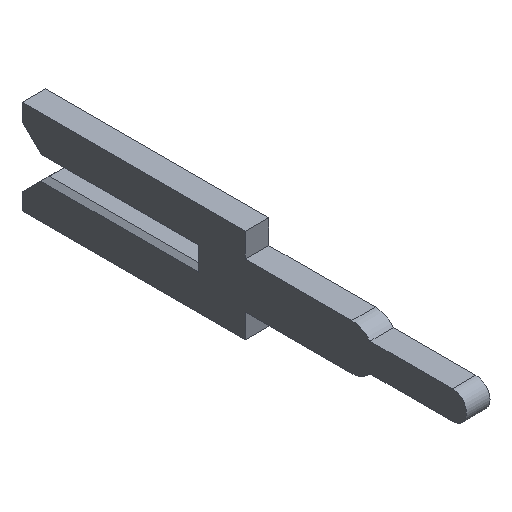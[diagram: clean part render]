
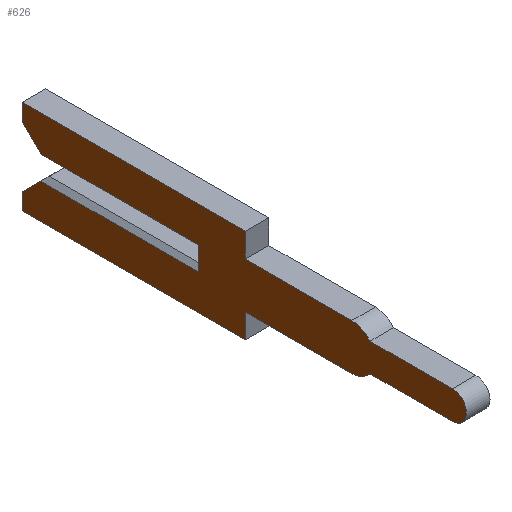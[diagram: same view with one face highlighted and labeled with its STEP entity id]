
A CAD part, isometric view. The second image highlights one B-rep face of the part: STEP entity #626.
In plain terms, the highlighted planar face has unit normal (-1, 0, 0).
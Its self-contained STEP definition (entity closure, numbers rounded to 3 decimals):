
#2 = VERTEX_POINT ( 'NONE', #481 ) ;
#6 = PLANE ( 'NONE',  #403 ) ;
#7 = VERTEX_POINT ( 'NONE', #49 ) ;
#17 = EDGE_CURVE ( 'NONE', #131, #633, #643, .T. ) ;
#24 = VECTOR ( 'NONE', #287, 1000. ) ;
#26 = DIRECTION ( 'NONE',  ( 0., 0., -1. ) ) ;
#46 = VERTEX_POINT ( 'NONE', #367 ) ;
#49 = CARTESIAN_POINT ( 'NONE',  ( -0.254, -3.705, 0.305 ) ) ;
#50 = EDGE_CURVE ( 'NONE', #881, #320, #313, .T. ) ;
#56 = LINE ( 'NONE', #779, #269 ) ;
#57 = CARTESIAN_POINT ( 'NONE',  ( -0.254, -3.315, 0.495 ) ) ;
#60 = CARTESIAN_POINT ( 'NONE',  ( -0.254, -1.016, 1.016 ) ) ;
#68 = CARTESIAN_POINT ( 'NONE',  ( -0.254, -5.486, -0.305 ) ) ;
#69 = ORIENTED_EDGE ( 'NONE', *, *, #948, .F. ) ;
#78 = LINE ( 'NONE', #391, #757 ) ;
#83 = CARTESIAN_POINT ( 'NONE',  ( -0.254, -5.486, 0. ) ) ;
#84 = CARTESIAN_POINT ( 'NONE',  ( -0.254, -1.016, 0.495 ) ) ;
#89 = DIRECTION ( 'NONE',  ( 0., -1., 0. ) ) ;
#98 = DIRECTION ( 'NONE',  ( 0., 0., -1. ) ) ;
#101 = CARTESIAN_POINT ( 'NONE',  ( -0.254, 3.404, 0.254 ) ) ;
#110 = ORIENTED_EDGE ( 'NONE', *, *, #730, .T. ) ;
#122 = VECTOR ( 'NONE', #89, 1000. ) ;
#126 = VECTOR ( 'NONE', #219, 1000. ) ;
#127 = DIRECTION ( 'NONE',  ( 0., 0., -1. ) ) ;
#131 = VERTEX_POINT ( 'NONE', #675 ) ;
#138 = DIRECTION ( 'NONE',  ( 0., -1., 0. ) ) ;
#141 = EDGE_CURVE ( 'NONE', #320, #7, #536, .T. ) ;
#144 = CARTESIAN_POINT ( 'NONE',  ( -0.254, -1.016, -0.495 ) ) ;
#148 = CARTESIAN_POINT ( 'NONE',  ( -0.254, -1.016, 0.495 ) ) ;
#166 = CARTESIAN_POINT ( 'NONE',  ( -0.254, -3.315, 0. ) ) ;
#170 = CARTESIAN_POINT ( 'NONE',  ( -0.254, -5.486, 0.305 ) ) ;
#187 = ORIENTED_EDGE ( 'NONE', *, *, #50, .F. ) ;
#190 = EDGE_CURVE ( 'NONE', #2, #390, #788, .T. ) ;
#194 = DIRECTION ( 'NONE',  ( 1., 0., 0. ) ) ;
#198 = VECTOR ( 'NONE', #433, 1000. ) ;
#208 = CARTESIAN_POINT ( 'NONE',  ( -0.254, 3.315, -0.165 ) ) ;
#217 = VERTEX_POINT ( 'NONE', #337 ) ;
#218 = CARTESIAN_POINT ( 'NONE',  ( -0.254, -3.315, -0.495 ) ) ;
#219 = DIRECTION ( 'NONE',  ( 0., -0.707, 0.707 ) ) ;
#224 = DIRECTION ( 'NONE',  ( 1., 0., 0. ) ) ;
#226 = FACE_OUTER_BOUND ( 'NONE', #593, .T. ) ;
#232 = LINE ( 'NONE', #710, #659 ) ;
#240 = VECTOR ( 'NONE', #402, 1000. ) ;
#249 = LINE ( 'NONE', #588, #342 ) ;
#260 = CARTESIAN_POINT ( 'NONE',  ( -0.254, 3.81, 1.016 ) ) ;
#263 = DIRECTION ( 'NONE',  ( 0., 1., 0. ) ) ;
#268 = VECTOR ( 'NONE', #519, 1000. ) ;
#269 = VECTOR ( 'NONE', #745, 1000. ) ;
#275 = VECTOR ( 'NONE', #938, 1000. ) ;
#282 = CARTESIAN_POINT ( 'NONE',  ( -0.254, 3.81, 1.016 ) ) ;
#287 = DIRECTION ( 'NONE',  ( 0., 1., 0. ) ) ;
#300 = DIRECTION ( 'NONE',  ( 0., -1., 0. ) ) ;
#303 = ORIENTED_EDGE ( 'NONE', *, *, #17, .F. ) ;
#304 = ORIENTED_EDGE ( 'NONE', *, *, #783, .F. ) ;
#305 = CARTESIAN_POINT ( 'NONE',  ( -0.254, -1.016, 1.016 ) ) ;
#312 = EDGE_CURVE ( 'NONE', #498, #881, #691, .T. ) ;
#313 = LINE ( 'NONE', #148, #952 ) ;
#320 = VERTEX_POINT ( 'NONE', #57 ) ;
#325 = CARTESIAN_POINT ( 'NONE',  ( -0.254, -3.315, 0.305 ) ) ;
#331 = EDGE_CURVE ( 'NONE', #633, #217, #763, .T. ) ;
#337 = CARTESIAN_POINT ( 'NONE',  ( -0.254, 3.404, -0.254 ) ) ;
#342 = VECTOR ( 'NONE', #592, 1000. ) ;
#343 = CARTESIAN_POINT ( 'NONE',  ( -0.254, -3.315, 0. ) ) ;
#344 = AXIS2_PLACEMENT_3D ( 'NONE', #343, #194, #127 ) ;
#367 = CARTESIAN_POINT ( 'NONE',  ( -0.254, -3.705, -0.305 ) ) ;
#388 = CARTESIAN_POINT ( 'NONE',  ( -0.254, -3.315, -0.254 ) ) ;
#390 = VERTEX_POINT ( 'NONE', #260 ) ;
#391 = CARTESIAN_POINT ( 'NONE',  ( -0.254, -1.016, -1.016 ) ) ;
#394 = LINE ( 'NONE', #282, #652 ) ;
#399 = EDGE_CURVE ( 'NONE', #858, #131, #232, .T. ) ;
#402 = DIRECTION ( 'NONE',  ( 0., -1., 0. ) ) ;
#403 = AXIS2_PLACEMENT_3D ( 'NONE', #166, #545, #98 ) ;
#407 = ORIENTED_EDGE ( 'NONE', *, *, #141, .F. ) ;
#415 = CARTESIAN_POINT ( 'NONE',  ( -0.254, 3.81, -0.66 ) ) ;
#421 = CARTESIAN_POINT ( 'NONE',  ( -0.254, 3.81, 0.66 ) ) ;
#422 = ORIENTED_EDGE ( 'NONE', *, *, #190, .F. ) ;
#433 = DIRECTION ( 'NONE',  ( 0., 1., 0. ) ) ;
#445 = ORIENTED_EDGE ( 'NONE', *, *, #637, .F. ) ;
#459 = CARTESIAN_POINT ( 'NONE',  ( -0.254, 3.315, 0.165 ) ) ;
#463 = ORIENTED_EDGE ( 'NONE', *, *, #399, .F. ) ;
#473 = EDGE_CURVE ( 'NONE', #628, #726, #778, .T. ) ;
#481 = CARTESIAN_POINT ( 'NONE',  ( -0.254, 3.81, 0.66 ) ) ;
#498 = VERTEX_POINT ( 'NONE', #305 ) ;
#507 = CARTESIAN_POINT ( 'NONE',  ( -0.254, -3.315, -0.305 ) ) ;
#518 = ORIENTED_EDGE ( 'NONE', *, *, #703, .F. ) ;
#519 = DIRECTION ( 'NONE',  ( 0., 0.707, 0.707 ) ) ;
#536 = CIRCLE ( 'NONE', #344, 0.495 ) ;
#542 = LINE ( 'NONE', #459, #268 ) ;
#545 = DIRECTION ( 'NONE',  ( 1., 0., 0. ) ) ;
#551 = ORIENTED_EDGE ( 'NONE', *, *, #331, .F. ) ;
#558 = DIRECTION ( 'NONE',  ( 0., 0., 1. ) ) ;
#586 = ORIENTED_EDGE ( 'NONE', *, *, #665, .F. ) ;
#588 = CARTESIAN_POINT ( 'NONE',  ( -0.254, 3.81, 0.254 ) ) ;
#592 = DIRECTION ( 'NONE',  ( 0., -1., 0. ) ) ;
#593 = EDGE_LOOP ( 'NONE', ( #69, #639, #744, #445, #407, #187, #846, #518, #422, #812, #110, #586, #946, #551, #303, #463, #677, #304 ) ) ;
#599 = EDGE_CURVE ( 'NONE', #217, #826, #829, .T. ) ;
#611 = AXIS2_PLACEMENT_3D ( 'NONE', #83, #224, #750 ) ;
#618 = LINE ( 'NONE', #507, #24 ) ;
#620 = AXIS2_PLACEMENT_3D ( 'NONE', #903, #766, #760 ) ;
#626 = ADVANCED_FACE ( 'NONE', ( #226 ), #6, .F. ) ;
#628 = VERTEX_POINT ( 'NONE', #170 ) ;
#633 = VERTEX_POINT ( 'NONE', #775 ) ;
#637 = EDGE_CURVE ( 'NONE', #7, #628, #949, .T. ) ;
#639 = ORIENTED_EDGE ( 'NONE', *, *, #685, .F. ) ;
#643 = LINE ( 'NONE', #415, #932 ) ;
#652 = VECTOR ( 'NONE', #138, 1000. ) ;
#655 = EDGE_CURVE ( 'NONE', #666, #858, #78, .T. ) ;
#658 = VERTEX_POINT ( 'NONE', #843 ) ;
#659 = VECTOR ( 'NONE', #263, 1000. ) ;
#661 = CIRCLE ( 'NONE', #620, 0.495 ) ;
#665 = EDGE_CURVE ( 'NONE', #826, #658, #56, .T. ) ;
#666 = VERTEX_POINT ( 'NONE', #736 ) ;
#671 = VERTEX_POINT ( 'NONE', #101 ) ;
#675 = CARTESIAN_POINT ( 'NONE',  ( -0.254, 3.81, -1.016 ) ) ;
#677 = ORIENTED_EDGE ( 'NONE', *, *, #655, .F. ) ;
#685 = EDGE_CURVE ( 'NONE', #726, #46, #618, .T. ) ;
#691 = LINE ( 'NONE', #60, #862 ) ;
#703 = EDGE_CURVE ( 'NONE', #390, #498, #394, .T. ) ;
#710 = CARTESIAN_POINT ( 'NONE',  ( -0.254, 3.81, -1.016 ) ) ;
#726 = VERTEX_POINT ( 'NONE', #68 ) ;
#730 = EDGE_CURVE ( 'NONE', #671, #658, #249, .T. ) ;
#731 = CARTESIAN_POINT ( 'NONE',  ( -0.254, -1.016, -1.016 ) ) ;
#736 = CARTESIAN_POINT ( 'NONE',  ( -0.254, -1.016, -0.495 ) ) ;
#740 = CARTESIAN_POINT ( 'NONE',  ( -0.254, 0., -0.254 ) ) ;
#744 = ORIENTED_EDGE ( 'NONE', *, *, #473, .F. ) ;
#745 = DIRECTION ( 'NONE',  ( 0., 0., 1. ) ) ;
#750 = DIRECTION ( 'NONE',  ( 0., 0., -1. ) ) ;
#757 = VECTOR ( 'NONE', #26, 1000. ) ;
#760 = DIRECTION ( 'NONE',  ( 0., 0., -1. ) ) ;
#763 = LINE ( 'NONE', #208, #126 ) ;
#766 = DIRECTION ( 'NONE',  ( 1., 0., 0. ) ) ;
#775 = CARTESIAN_POINT ( 'NONE',  ( -0.254, 3.81, -0.66 ) ) ;
#778 = CIRCLE ( 'NONE', #611, 0.305 ) ;
#779 = CARTESIAN_POINT ( 'NONE',  ( -0.254, 0., 0.165 ) ) ;
#783 = EDGE_CURVE ( 'NONE', #800, #666, #853, .T. ) ;
#788 = LINE ( 'NONE', #421, #275 ) ;
#800 = VERTEX_POINT ( 'NONE', #218 ) ;
#806 = DIRECTION ( 'NONE',  ( 0., 0., -1. ) ) ;
#812 = ORIENTED_EDGE ( 'NONE', *, *, #931, .F. ) ;
#826 = VERTEX_POINT ( 'NONE', #740 ) ;
#829 = LINE ( 'NONE', #388, #122 ) ;
#843 = CARTESIAN_POINT ( 'NONE',  ( -0.254, 0., 0.254 ) ) ;
#846 = ORIENTED_EDGE ( 'NONE', *, *, #312, .F. ) ;
#853 = LINE ( 'NONE', #144, #198 ) ;
#858 = VERTEX_POINT ( 'NONE', #731 ) ;
#862 = VECTOR ( 'NONE', #806, 1000. ) ;
#881 = VERTEX_POINT ( 'NONE', #84 ) ;
#903 = CARTESIAN_POINT ( 'NONE',  ( -0.254, -3.315, 0. ) ) ;
#931 = EDGE_CURVE ( 'NONE', #671, #2, #542, .T. ) ;
#932 = VECTOR ( 'NONE', #558, 1000. ) ;
#938 = DIRECTION ( 'NONE',  ( 0., 0., 1. ) ) ;
#946 = ORIENTED_EDGE ( 'NONE', *, *, #599, .F. ) ;
#948 = EDGE_CURVE ( 'NONE', #46, #800, #661, .T. ) ;
#949 = LINE ( 'NONE', #325, #240 ) ;
#952 = VECTOR ( 'NONE', #300, 1000. ) ;
